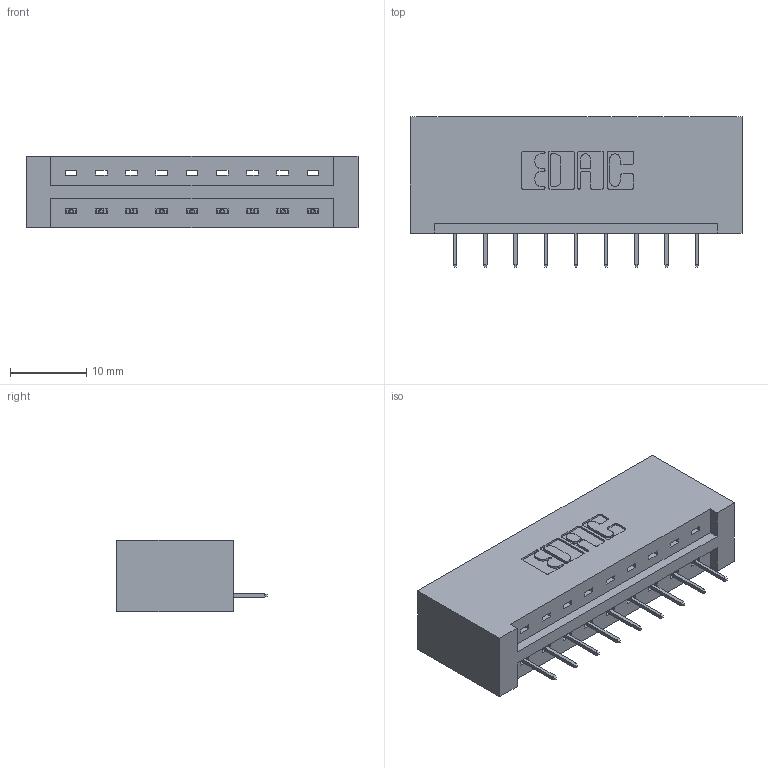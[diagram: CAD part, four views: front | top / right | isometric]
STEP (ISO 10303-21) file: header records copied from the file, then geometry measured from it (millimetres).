
FILE_DESCRIPTION (( 'STEP AP203' ), '1' );
FILE_NAME ('387-009-524-101.STEP', '2018-09-10T05:29:07', ( '' ), ( '' ), 'SwSTEP 2.0', 'SolidWorks 2016', '' );
FILE_SCHEMA (( 'CONFIG_CONTROL_DESIGN' ));
Length unit declared in the file: inch
Products named in the file (3): 337 Part_No Mounting Lugs; 345-292-001_345-293-124; 387-009-524-101
Assembly tree (10 placements, depth 2):
  387-009-524-101
    337 Part_No Mounting Lugs
    345-292-001_345-293-124  x9
Bounding box: 43.54 x 19.69 x 9.4 mm (x, y, z)
Volume: 4815 mm3; surface area: 4648.8 mm2
Topology: 10 solids, 10 shells, 700 faces, 2015 edges, 1306 vertices
Faces by surface type: plane 534, cylinder 166
Entity records: 10755 total; most frequent: CARTESIAN_POINT 1877, ORIENTED_EDGE 1822, DIRECTION 1641, EDGE_CURVE 911, LINE 795, VECTOR 795, VERTEX_POINT 602, AXIS2_PLACEMENT_3D 423
